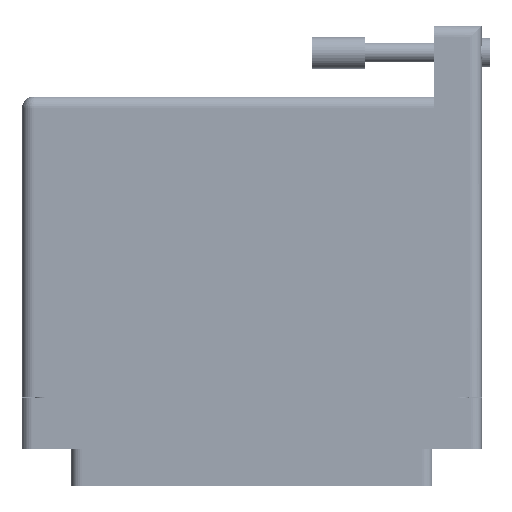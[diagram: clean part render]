
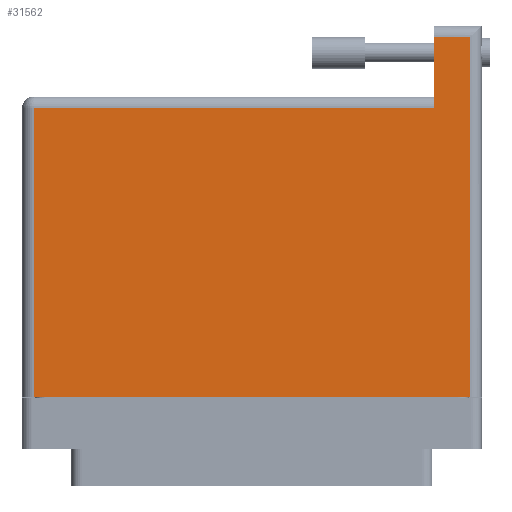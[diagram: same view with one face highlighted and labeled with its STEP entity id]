
A CAD part, front view. The second image highlights one B-rep face of the part: STEP entity #31562.
In plain terms, the highlighted face is planar.
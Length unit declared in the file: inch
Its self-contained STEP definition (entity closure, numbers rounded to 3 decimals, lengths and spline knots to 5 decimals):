
#1055 = DIRECTION ( 'NONE',  ( 0., 1., 0. ) ) ;
#1647 = VECTOR ( 'NONE', #1055, 39.37008 ) ;
#3445 = VECTOR ( 'NONE', #58485, 39.37008 ) ;
#4345 = CARTESIAN_POINT ( 'NONE',  ( -1.359, 1.675, 0.617 ) ) ;
#4538 = CARTESIAN_POINT ( 'NONE',  ( -1.359, 1.605, 0.617 ) ) ;
#5815 = ORIENTED_EDGE ( 'NONE', *, *, #19043, .T. ) ;
#6554 = CARTESIAN_POINT ( 'NONE',  ( 1.289, 2.095, 0.617 ) ) ;
#6635 = EDGE_LOOP ( 'NONE', ( #5815, #52663, #27247, #16524, #58159, #15217 ) ) ;
#7871 = LINE ( 'NONE', #20729, #56867 ) ;
#14812 = PLANE ( 'NONE',  #54905 ) ;
#15217 = ORIENTED_EDGE ( 'NONE', *, *, #37968, .T. ) ;
#15300 = VERTEX_POINT ( 'NONE', #22190 ) ;
#15901 = EDGE_CURVE ( 'NONE', #65315, #65358, #16828, .T. ) ;
#16524 = ORIENTED_EDGE ( 'NONE', *, *, #15901, .T. ) ;
#16828 = LINE ( 'NONE', #6554, #1647 ) ;
#17102 = FACE_OUTER_BOUND ( 'NONE', #6635, .T. ) ;
#19043 = EDGE_CURVE ( 'NONE', #64945, #19623, #24378, .T. ) ;
#19623 = VERTEX_POINT ( 'NONE', #73086 ) ;
#20466 = DIRECTION ( 'NONE',  ( 1., 0., 0. ) ) ;
#20729 = CARTESIAN_POINT ( 'NONE',  ( -1.359, -0.1, 0.617 ) ) ;
#20785 = VECTOR ( 'NONE', #23002, 39.37008 ) ;
#22190 = CARTESIAN_POINT ( 'NONE',  ( -1.289, -0.1, 0.617 ) ) ;
#23002 = DIRECTION ( 'NONE',  ( -1., 0., 0. ) ) ;
#24378 = LINE ( 'NONE', #4538, #20785 ) ;
#27247 = ORIENTED_EDGE ( 'NONE', *, *, #33397, .T. ) ;
#31038 = LINE ( 'NONE', #63897, #33695 ) ;
#31562 = ADVANCED_FACE ( 'NONE', ( #17102 ), #14812, .F. ) ;
#32177 = DIRECTION ( 'NONE',  ( -1., 0., 0. ) ) ;
#33397 = EDGE_CURVE ( 'NONE', #15300, #65315, #7871, .T. ) ;
#33695 = VECTOR ( 'NONE', #40835, 39.37008 ) ;
#37156 = CARTESIAN_POINT ( 'NONE',  ( -1.359, 2.025, 0.617 ) ) ;
#37440 = VECTOR ( 'NONE', #42403, 39.37008 ) ;
#37463 = DIRECTION ( 'NONE',  ( 0., 0., -1. ) ) ;
#37912 = EDGE_CURVE ( 'NONE', #19623, #15300, #58612, .T. ) ;
#37968 = EDGE_CURVE ( 'NONE', #71454, #64945, #31038, .T. ) ;
#39527 = CARTESIAN_POINT ( 'NONE',  ( 1.079, 2.025, 0.617 ) ) ;
#40835 = DIRECTION ( 'NONE',  ( 0., -1., 0. ) ) ;
#42403 = DIRECTION ( 'NONE',  ( -1., 0., 0. ) ) ;
#43943 = CARTESIAN_POINT ( 'NONE',  ( 1.289, -0.1, 0.617 ) ) ;
#44952 = CARTESIAN_POINT ( 'NONE',  ( 1.079, 1.605, 0.617 ) ) ;
#46302 = CARTESIAN_POINT ( 'NONE',  ( -1.289, -0.1, 0.617 ) ) ;
#51656 = LINE ( 'NONE', #37156, #37440 ) ;
#52663 = ORIENTED_EDGE ( 'NONE', *, *, #37912, .T. ) ;
#53450 = EDGE_CURVE ( 'NONE', #65358, #71454, #51656, .T. ) ;
#54905 = AXIS2_PLACEMENT_3D ( 'NONE', #4345, #37463, #32177 ) ;
#56350 = CARTESIAN_POINT ( 'NONE',  ( 1.289, 2.025, 0.617 ) ) ;
#56867 = VECTOR ( 'NONE', #20466, 39.37008 ) ;
#58159 = ORIENTED_EDGE ( 'NONE', *, *, #53450, .T. ) ;
#58485 = DIRECTION ( 'NONE',  ( 0., -1., 0. ) ) ;
#58612 = LINE ( 'NONE', #46302, #3445 ) ;
#63897 = CARTESIAN_POINT ( 'NONE',  ( 1.079, 2.095, 0.617 ) ) ;
#64945 = VERTEX_POINT ( 'NONE', #44952 ) ;
#65315 = VERTEX_POINT ( 'NONE', #43943 ) ;
#65358 = VERTEX_POINT ( 'NONE', #56350 ) ;
#71454 = VERTEX_POINT ( 'NONE', #39527 ) ;
#73086 = CARTESIAN_POINT ( 'NONE',  ( -1.289, 1.605, 0.617 ) ) ;
